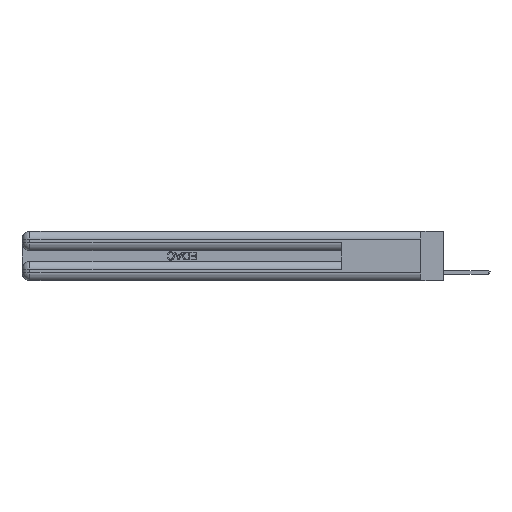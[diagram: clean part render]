
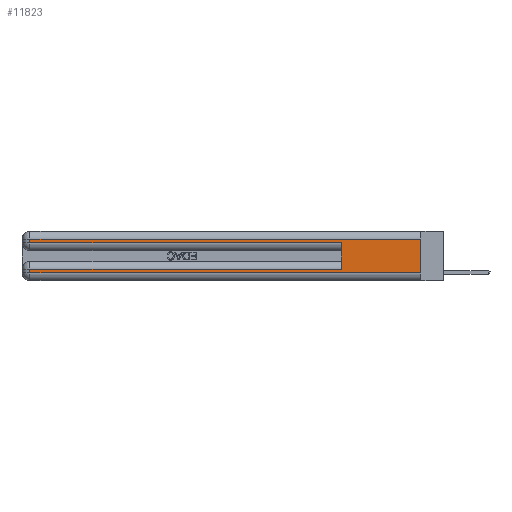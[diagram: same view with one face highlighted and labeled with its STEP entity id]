
A CAD part, left-side view. The second image highlights one B-rep face of the part: STEP entity #11823.
In plain terms, the highlighted planar face has unit normal (-1, 0, 0).
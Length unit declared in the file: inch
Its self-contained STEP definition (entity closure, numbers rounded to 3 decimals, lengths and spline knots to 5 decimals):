
#31 = ORIENTED_EDGE ( 'NONE', *, *, #30007, .F. ) ;
#890 = EDGE_LOOP ( 'NONE', ( #31, #30449, #30355, #32946, #16174, #33101, #8890, #3741 ) ) ;
#1479 = DIRECTION ( 'NONE',  ( 0., 0., -1. ) ) ;
#2234 = PLANE ( 'NONE',  #10655 ) ;
#2459 = CARTESIAN_POINT ( 'NONE',  ( 0., 0., 0.06 ) ) ;
#3166 = VECTOR ( 'NONE', #24552, 39.37008 ) ;
#3507 = VECTOR ( 'NONE', #30861, 39.37008 ) ;
#3741 = ORIENTED_EDGE ( 'NONE', *, *, #4982, .T. ) ;
#4728 = VECTOR ( 'NONE', #21019, 39.37008 ) ;
#4982 = EDGE_CURVE ( 'NONE', #18013, #12485, #22062, .T. ) ;
#5244 = CARTESIAN_POINT ( 'NONE',  ( 0., 2.94, 0.085 ) ) ;
#6293 = CARTESIAN_POINT ( 'NONE',  ( 0., 2.94, 0.285 ) ) ;
#6314 = VERTEX_POINT ( 'NONE', #6293 ) ;
#6428 = CARTESIAN_POINT ( 'NONE',  ( 0., 0.6, 0.285 ) ) ;
#6709 = LINE ( 'NONE', #30323, #3507 ) ;
#7301 = VERTEX_POINT ( 'NONE', #30927 ) ;
#7821 = VECTOR ( 'NONE', #1479, 39.37008 ) ;
#8246 = VERTEX_POINT ( 'NONE', #6428 ) ;
#8890 = ORIENTED_EDGE ( 'NONE', *, *, #15303, .T. ) ;
#8935 = VERTEX_POINT ( 'NONE', #16388 ) ;
#10006 = DIRECTION ( 'NONE',  ( 1., 0., 0. ) ) ;
#10655 = AXIS2_PLACEMENT_3D ( 'NONE', #18016, #10006, #33089 ) ;
#10788 = LINE ( 'NONE', #26160, #4728 ) ;
#11034 = VERTEX_POINT ( 'NONE', #5244 ) ;
#11038 = VECTOR ( 'NONE', #15144, 39.37008 ) ;
#11190 = VECTOR ( 'NONE', #19177, 39.37008 ) ;
#11525 = EDGE_CURVE ( 'NONE', #27064, #11034, #28351, .T. ) ;
#11823 = ADVANCED_FACE ( 'NONE', ( #19399 ), #2234, .F. ) ;
#12485 = VERTEX_POINT ( 'NONE', #17483 ) ;
#12564 = CARTESIAN_POINT ( 'NONE',  ( 0., 0., 0.085 ) ) ;
#13780 = LINE ( 'NONE', #19068, #29968 ) ;
#13910 = CARTESIAN_POINT ( 'NONE',  ( 0., 0., 0.285 ) ) ;
#15144 = DIRECTION ( 'NONE',  ( 0., 1., 0. ) ) ;
#15303 = EDGE_CURVE ( 'NONE', #11034, #18013, #10788, .T. ) ;
#16174 = ORIENTED_EDGE ( 'NONE', *, *, #26727, .F. ) ;
#16388 = CARTESIAN_POINT ( 'NONE',  ( 0., 0., 0.31 ) ) ;
#16811 = CARTESIAN_POINT ( 'NONE',  ( 0., 2.94, 0.37 ) ) ;
#17483 = CARTESIAN_POINT ( 'NONE',  ( 0., 0., 0.06 ) ) ;
#18013 = VERTEX_POINT ( 'NONE', #21607 ) ;
#18016 = CARTESIAN_POINT ( 'NONE',  ( 0., 0., 0.37 ) ) ;
#19068 = CARTESIAN_POINT ( 'NONE',  ( 0., 0., 0.37 ) ) ;
#19177 = DIRECTION ( 'NONE',  ( 0., -1., 0. ) ) ;
#19399 = FACE_OUTER_BOUND ( 'NONE', #890, .T. ) ;
#21019 = DIRECTION ( 'NONE',  ( 0., 0., -1. ) ) ;
#21164 = EDGE_CURVE ( 'NONE', #8935, #7301, #23647, .T. ) ;
#21607 = CARTESIAN_POINT ( 'NONE',  ( 0., 2.94, 0.06 ) ) ;
#21719 = EDGE_CURVE ( 'NONE', #6314, #8246, #28944, .T. ) ;
#21944 = CARTESIAN_POINT ( 'NONE',  ( 0., 0., 0.31 ) ) ;
#22062 = LINE ( 'NONE', #2459, #30208 ) ;
#23458 = LINE ( 'NONE', #16811, #7821 ) ;
#23647 = LINE ( 'NONE', #21944, #3166 ) ;
#24552 = DIRECTION ( 'NONE',  ( 0., 1., 0. ) ) ;
#25405 = DIRECTION ( 'NONE',  ( 0., -1., 0. ) ) ;
#26160 = CARTESIAN_POINT ( 'NONE',  ( 0., 2.94, 0.37 ) ) ;
#26525 = CARTESIAN_POINT ( 'NONE',  ( 0., 0.6, 0.085 ) ) ;
#26727 = EDGE_CURVE ( 'NONE', #27064, #8246, #6709, .T. ) ;
#27064 = VERTEX_POINT ( 'NONE', #26525 ) ;
#28351 = LINE ( 'NONE', #12564, #11038 ) ;
#28586 = EDGE_CURVE ( 'NONE', #7301, #6314, #23458, .T. ) ;
#28944 = LINE ( 'NONE', #13910, #11190 ) ;
#29533 = DIRECTION ( 'NONE',  ( 0., 0., -1. ) ) ;
#29968 = VECTOR ( 'NONE', #29533, 39.37008 ) ;
#30007 = EDGE_CURVE ( 'NONE', #8935, #12485, #13780, .T. ) ;
#30208 = VECTOR ( 'NONE', #25405, 39.37008 ) ;
#30323 = CARTESIAN_POINT ( 'NONE',  ( 0., 0.6, 0.145 ) ) ;
#30355 = ORIENTED_EDGE ( 'NONE', *, *, #28586, .T. ) ;
#30449 = ORIENTED_EDGE ( 'NONE', *, *, #21164, .T. ) ;
#30861 = DIRECTION ( 'NONE',  ( 0., 0., 1. ) ) ;
#30927 = CARTESIAN_POINT ( 'NONE',  ( 0., 2.94, 0.31 ) ) ;
#32946 = ORIENTED_EDGE ( 'NONE', *, *, #21719, .T. ) ;
#33089 = DIRECTION ( 'NONE',  ( 0., 0., -1. ) ) ;
#33101 = ORIENTED_EDGE ( 'NONE', *, *, #11525, .T. ) ;
